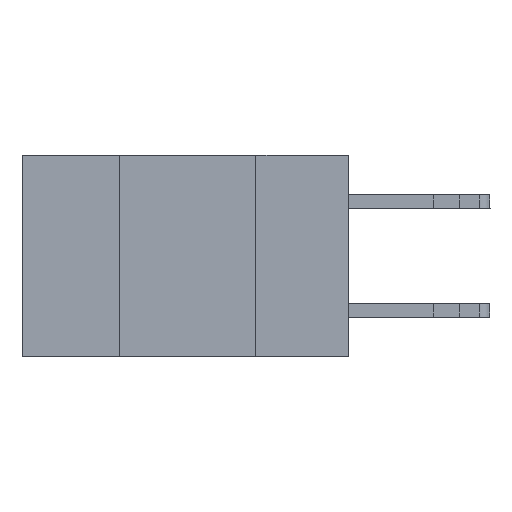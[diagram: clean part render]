
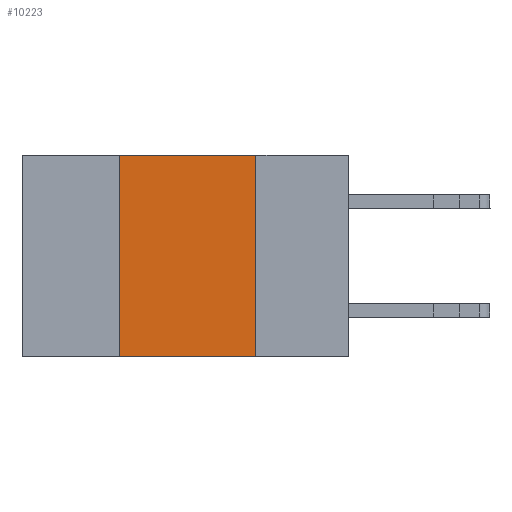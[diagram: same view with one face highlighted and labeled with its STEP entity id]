
A CAD part, left-side view. The second image highlights one B-rep face of the part: STEP entity #10223.
In plain terms, the highlighted planar face has unit normal (-1, 0, 0).
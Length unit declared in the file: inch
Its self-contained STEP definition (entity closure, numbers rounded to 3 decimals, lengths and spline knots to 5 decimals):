
#390 = LINE ( 'NONE', #6869, #19576 ) ;
#1056 = ORIENTED_EDGE ( 'NONE', *, *, #5673, .F. ) ;
#2280 = CARTESIAN_POINT ( 'NONE',  ( 0., 0.42, 0. ) ) ;
#2487 = LINE ( 'NONE', #7823, #10199 ) ;
#2552 = EDGE_CURVE ( 'NONE', #3766, #10272, #7938, .T. ) ;
#3597 = EDGE_CURVE ( 'NONE', #3766, #13917, #13314, .T. ) ;
#3766 = VERTEX_POINT ( 'NONE', #14054 ) ;
#4764 = VECTOR ( 'NONE', #7709, 39.37008 ) ;
#5175 = ORIENTED_EDGE ( 'NONE', *, *, #9052, .F. ) ;
#5672 = CARTESIAN_POINT ( 'NONE',  ( 0., 0.17, 0. ) ) ;
#5673 = EDGE_CURVE ( 'NONE', #6006, #10272, #2487, .T. ) ;
#6006 = VERTEX_POINT ( 'NONE', #5672 ) ;
#6869 = CARTESIAN_POINT ( 'NONE',  ( 0., 0.6, 0. ) ) ;
#6930 = DIRECTION ( 'NONE',  ( 0., -1., 0. ) ) ;
#7709 = DIRECTION ( 'NONE',  ( 0., 0., 1. ) ) ;
#7823 = CARTESIAN_POINT ( 'NONE',  ( 0., 0.17, 0. ) ) ;
#7938 = LINE ( 'NONE', #8552, #8406 ) ;
#8206 = CARTESIAN_POINT ( 'NONE',  ( 0., 0.6, 0. ) ) ;
#8345 = CARTESIAN_POINT ( 'NONE',  ( 0., 0.17, -0.37 ) ) ;
#8406 = VECTOR ( 'NONE', #8684, 39.37008 ) ;
#8552 = CARTESIAN_POINT ( 'NONE',  ( 0., 0.6, -0.37 ) ) ;
#8684 = DIRECTION ( 'NONE',  ( 0., -1., 0. ) ) ;
#9052 = EDGE_CURVE ( 'NONE', #13917, #6006, #390, .T. ) ;
#9340 = DIRECTION ( 'NONE',  ( 0., 0., -1. ) ) ;
#9754 = DIRECTION ( 'NONE',  ( 0., 0., -1. ) ) ;
#10199 = VECTOR ( 'NONE', #9340, 39.37008 ) ;
#10223 = ADVANCED_FACE ( 'NONE', ( #18210 ), #15706, .F. ) ;
#10272 = VERTEX_POINT ( 'NONE', #8345 ) ;
#10348 = EDGE_LOOP ( 'NONE', ( #1056, #5175, #13245, #13704 ) ) ;
#10757 = CARTESIAN_POINT ( 'NONE',  ( 0., 0.42, 0. ) ) ;
#10767 = AXIS2_PLACEMENT_3D ( 'NONE', #8206, #18664, #9754 ) ;
#13245 = ORIENTED_EDGE ( 'NONE', *, *, #3597, .F. ) ;
#13314 = LINE ( 'NONE', #10757, #4764 ) ;
#13704 = ORIENTED_EDGE ( 'NONE', *, *, #2552, .T. ) ;
#13917 = VERTEX_POINT ( 'NONE', #2280 ) ;
#14054 = CARTESIAN_POINT ( 'NONE',  ( 0., 0.42, -0.37 ) ) ;
#15706 = PLANE ( 'NONE',  #10767 ) ;
#18210 = FACE_OUTER_BOUND ( 'NONE', #10348, .T. ) ;
#18664 = DIRECTION ( 'NONE',  ( 1., 0., 0. ) ) ;
#19576 = VECTOR ( 'NONE', #6930, 39.37008 ) ;
